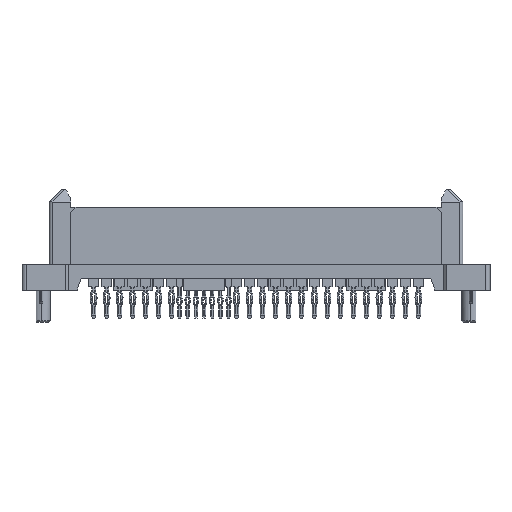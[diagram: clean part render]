
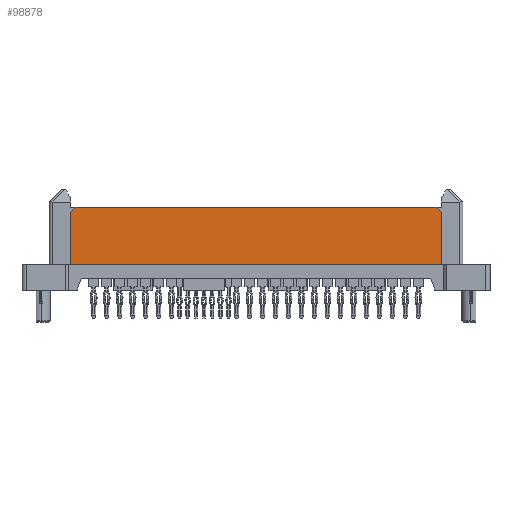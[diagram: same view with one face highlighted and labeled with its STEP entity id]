
A CAD part, top view. The second image highlights one B-rep face of the part: STEP entity #98878.
In plain terms, the highlighted planar face has unit normal (0, 0, 1).
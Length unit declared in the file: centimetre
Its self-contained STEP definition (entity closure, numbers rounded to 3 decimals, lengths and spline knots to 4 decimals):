
#4024 = VECTOR ( 'NONE', #44926, 100. ) ;
#5258 = DIRECTION ( 'NONE',  ( 0., 0., 1. ) ) ;
#6754 = LINE ( 'NONE', #16698, #119205 ) ;
#9192 = EDGE_CURVE ( 'NONE', #102789, #100642, #26383, .T. ) ;
#12898 = VECTOR ( 'NONE', #64293, 100. ) ;
#16698 = CARTESIAN_POINT ( 'NONE',  ( 1.8095, 0.535, 0.1825 ) ) ;
#17291 = CARTESIAN_POINT ( 'NONE',  ( -1.8095, 0.255, 0.1825 ) ) ;
#26383 = LINE ( 'NONE', #27665, #12898 ) ;
#26418 = VERTEX_POINT ( 'NONE', #17291 ) ;
#27665 = CARTESIAN_POINT ( 'NONE',  ( 0., 0.815, 0.1825 ) ) ;
#28168 = DIRECTION ( 'NONE',  ( 1., 0., 0. ) ) ;
#29278 = CARTESIAN_POINT ( 'NONE',  ( 1.8095, 0.255, 0.1825 ) ) ;
#29819 = ORIENTED_EDGE ( 'NONE', *, *, #78204, .T. ) ;
#30872 = DIRECTION ( 'NONE',  ( -0.707, 0.707, 0. ) ) ;
#32079 = VERTEX_POINT ( 'NONE', #74200 ) ;
#32095 = LINE ( 'NONE', #69945, #103413 ) ;
#35648 = LINE ( 'NONE', #110128, #4024 ) ;
#37832 = EDGE_CURVE ( 'NONE', #26418, #114413, #35648, .T. ) ;
#38129 = AXIS2_PLACEMENT_3D ( 'NONE', #113236, #5258, #28168 ) ;
#43512 = CARTESIAN_POINT ( 'NONE',  ( 1.7595, 0.815, 0.1825 ) ) ;
#43909 = EDGE_CURVE ( 'NONE', #100642, #32079, #63835, .T. ) ;
#44763 = LINE ( 'NONE', #55941, #96258 ) ;
#44926 = DIRECTION ( 'NONE',  ( 1., 0., 0. ) ) ;
#45822 = DIRECTION ( 'NONE',  ( -0.707, -0.707, 0. ) ) ;
#46824 = FACE_OUTER_BOUND ( 'NONE', #84442, .T. ) ;
#49892 = ORIENTED_EDGE ( 'NONE', *, *, #9192, .T. ) ;
#51815 = ORIENTED_EDGE ( 'NONE', *, *, #43909, .T. ) ;
#55941 = CARTESIAN_POINT ( 'NONE',  ( -1.8095, 0.535, 0.1825 ) ) ;
#63374 = DIRECTION ( 'NONE',  ( 0., 1., 0. ) ) ;
#63835 = LINE ( 'NONE', #93621, #99677 ) ;
#64293 = DIRECTION ( 'NONE',  ( -1., 0., 0. ) ) ;
#64960 = ORIENTED_EDGE ( 'NONE', *, *, #70296, .T. ) ;
#66468 = CARTESIAN_POINT ( 'NONE',  ( 1.8095, 0.765, 0.1825 ) ) ;
#69945 = CARTESIAN_POINT ( 'NONE',  ( 1.8095, 0.765, 0.1825 ) ) ;
#70296 = EDGE_CURVE ( 'NONE', #32079, #26418, #44763, .T. ) ;
#74200 = CARTESIAN_POINT ( 'NONE',  ( -1.8095, 0.765, 0.1825 ) ) ;
#76719 = EDGE_CURVE ( 'NONE', #84394, #102789, #32095, .T. ) ;
#78204 = EDGE_CURVE ( 'NONE', #114413, #84394, #6754, .T. ) ;
#84394 = VERTEX_POINT ( 'NONE', #66468 ) ;
#84442 = EDGE_LOOP ( 'NONE', ( #49892, #51815, #64960, #93195, #29819, #85000 ) ) ;
#85000 = ORIENTED_EDGE ( 'NONE', *, *, #76719, .T. ) ;
#93195 = ORIENTED_EDGE ( 'NONE', *, *, #37832, .T. ) ;
#93621 = CARTESIAN_POINT ( 'NONE',  ( -1.7595, 0.815, 0.1825 ) ) ;
#96258 = VECTOR ( 'NONE', #101294, 100. ) ;
#98878 = ADVANCED_FACE ( 'NONE', ( #46824 ), #99781, .T. ) ;
#99677 = VECTOR ( 'NONE', #45822, 100. ) ;
#99781 = PLANE ( 'NONE',  #38129 ) ;
#100642 = VERTEX_POINT ( 'NONE', #118729 ) ;
#101294 = DIRECTION ( 'NONE',  ( 0., -1., 0. ) ) ;
#102789 = VERTEX_POINT ( 'NONE', #43512 ) ;
#103413 = VECTOR ( 'NONE', #30872, 100. ) ;
#110128 = CARTESIAN_POINT ( 'NONE',  ( 0., 0.255, 0.1825 ) ) ;
#113236 = CARTESIAN_POINT ( 'NONE',  ( 0., 0.535, 0.1825 ) ) ;
#114413 = VERTEX_POINT ( 'NONE', #29278 ) ;
#118729 = CARTESIAN_POINT ( 'NONE',  ( -1.7595, 0.815, 0.1825 ) ) ;
#119205 = VECTOR ( 'NONE', #63374, 100. ) ;
